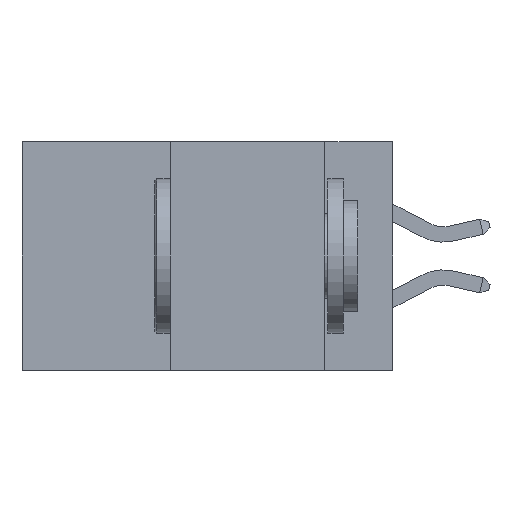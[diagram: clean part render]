
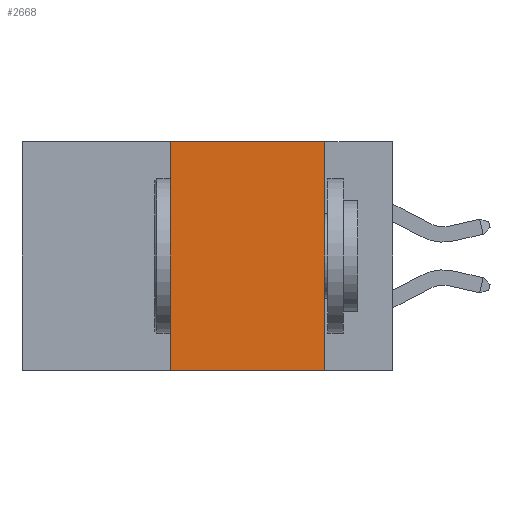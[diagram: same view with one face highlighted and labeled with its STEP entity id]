
A CAD part, left-side view. The second image highlights one B-rep face of the part: STEP entity #2668.
In plain terms, the highlighted planar face has unit normal (-1, 0, 0).
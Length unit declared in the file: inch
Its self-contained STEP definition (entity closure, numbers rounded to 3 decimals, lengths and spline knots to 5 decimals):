
#318 = EDGE_CURVE ( 'NONE', #6090, #7256, #25032, .T. ) ;
#2350 = CARTESIAN_POINT ( 'NONE',  ( 0., 0.36, 0. ) ) ;
#2668 = ADVANCED_FACE ( 'NONE', ( #3341 ), #20919, .F. ) ;
#3341 = FACE_OUTER_BOUND ( 'NONE', #14113, .T. ) ;
#3531 = ORIENTED_EDGE ( 'NONE', *, *, #9624, .F. ) ;
#4556 = EDGE_CURVE ( 'NONE', #23752, #7256, #21763, .T. ) ;
#6090 = VERTEX_POINT ( 'NONE', #21315 ) ;
#7256 = VERTEX_POINT ( 'NONE', #11076 ) ;
#7627 = ORIENTED_EDGE ( 'NONE', *, *, #318, .F. ) ;
#8266 = DIRECTION ( 'NONE',  ( 0., -1., 0. ) ) ;
#9624 = EDGE_CURVE ( 'NONE', #23701, #6090, #22891, .T. ) ;
#10131 = ORIENTED_EDGE ( 'NONE', *, *, #4556, .T. ) ;
#10254 = LINE ( 'NONE', #16520, #25685 ) ;
#11076 = CARTESIAN_POINT ( 'NONE',  ( 0., 0.11, -0.37 ) ) ;
#12228 = CARTESIAN_POINT ( 'NONE',  ( 0., 0.6, 0. ) ) ;
#13709 = VECTOR ( 'NONE', #15881, 39.37008 ) ;
#14113 = EDGE_LOOP ( 'NONE', ( #7627, #3531, #14876, #10131 ) ) ;
#14742 = CARTESIAN_POINT ( 'NONE',  ( 0., 0.6, -0.37 ) ) ;
#14843 = DIRECTION ( 'NONE',  ( 0., -1., 0. ) ) ;
#14876 = ORIENTED_EDGE ( 'NONE', *, *, #20474, .F. ) ;
#15881 = DIRECTION ( 'NONE',  ( 0., 0., -1. ) ) ;
#15997 = CARTESIAN_POINT ( 'NONE',  ( 0., 0.11, 0. ) ) ;
#16520 = CARTESIAN_POINT ( 'NONE',  ( 0., 0.36, 0. ) ) ;
#16604 = DIRECTION ( 'NONE',  ( 0., 0., 1. ) ) ;
#17534 = VECTOR ( 'NONE', #8266, 39.37008 ) ;
#18191 = DIRECTION ( 'NONE',  ( 0., 0., -1. ) ) ;
#18486 = AXIS2_PLACEMENT_3D ( 'NONE', #20629, #20748, #18191 ) ;
#20474 = EDGE_CURVE ( 'NONE', #23752, #23701, #10254, .T. ) ;
#20629 = CARTESIAN_POINT ( 'NONE',  ( 0., 0.6, 0. ) ) ;
#20737 = CARTESIAN_POINT ( 'NONE',  ( 0., 0.36, -0.37 ) ) ;
#20748 = DIRECTION ( 'NONE',  ( 1., 0., 0. ) ) ;
#20919 = PLANE ( 'NONE',  #18486 ) ;
#21315 = CARTESIAN_POINT ( 'NONE',  ( 0., 0.11, 0. ) ) ;
#21763 = LINE ( 'NONE', #14742, #25589 ) ;
#22891 = LINE ( 'NONE', #12228, #17534 ) ;
#23701 = VERTEX_POINT ( 'NONE', #2350 ) ;
#23752 = VERTEX_POINT ( 'NONE', #20737 ) ;
#25032 = LINE ( 'NONE', #15997, #13709 ) ;
#25589 = VECTOR ( 'NONE', #14843, 39.37008 ) ;
#25685 = VECTOR ( 'NONE', #16604, 39.37008 ) ;
